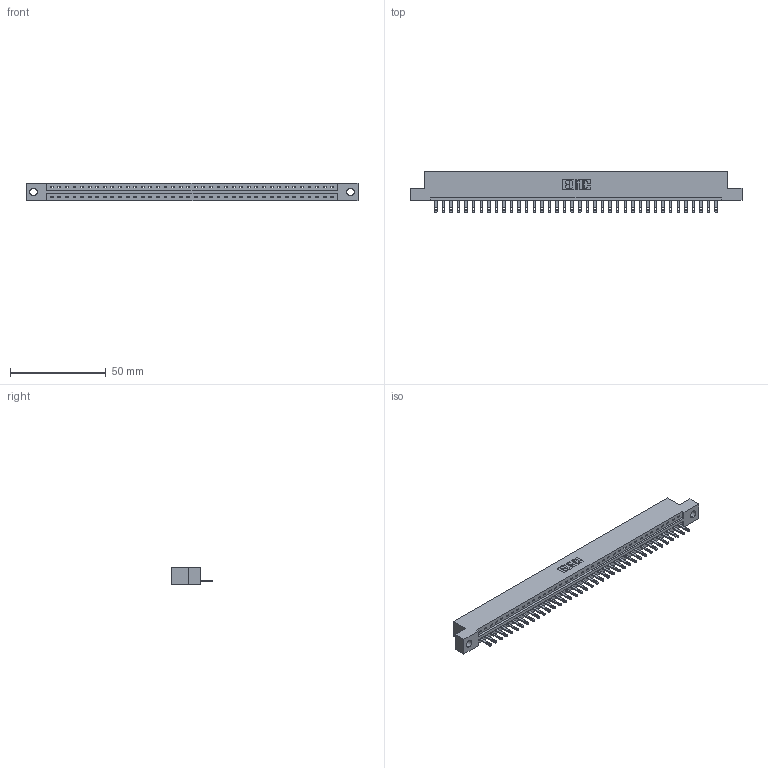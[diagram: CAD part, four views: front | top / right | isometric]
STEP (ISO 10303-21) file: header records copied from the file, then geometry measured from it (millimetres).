
FILE_DESCRIPTION (( 'STEP AP203' ), '1' );
FILE_NAME ('837-038-500-104.STEP', '2021-08-04T14:12:00', ( '' ), ( '' ), 'SwSTEP 2.0', 'SolidWorks 2020', '' );
FILE_SCHEMA (( 'CONFIG_CONTROL_DESIGN' ));
Length unit declared in the file: inch
Products named in the file (3): 345-292-001_345-293-100; 837-038-500-104; 837 Part_Flush Mounting Lugs - 0.156 Dia-TH
Assembly tree (39 placements, depth 2):
  837-038-500-104
    837 Part_Flush Mounting Lugs - 0.156 Dia-TH
    345-292-001_345-293-100  x38
Bounding box: 173.58 x 21.85 x 9.4 mm (x, y, z)
Volume: 17926.7 mm3; surface area: 18386.4 mm2
Topology: 39 solids, 39 shells, 2318 faces, 7151 edges, 4766 vertices
Faces by surface type: plane 1590, cylinder 728
Entity records: 28697 total; most frequent: CARTESIAN_POINT 5004, ORIENTED_EDGE 4978, DIRECTION 4221, EDGE_CURVE 2489, VECTOR 2357, LINE 2357, VERTEX_POINT 1658, AXIS2_PLACEMENT_3D 932
